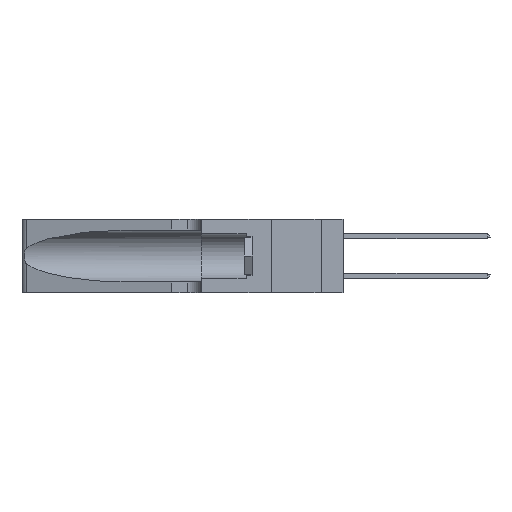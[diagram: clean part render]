
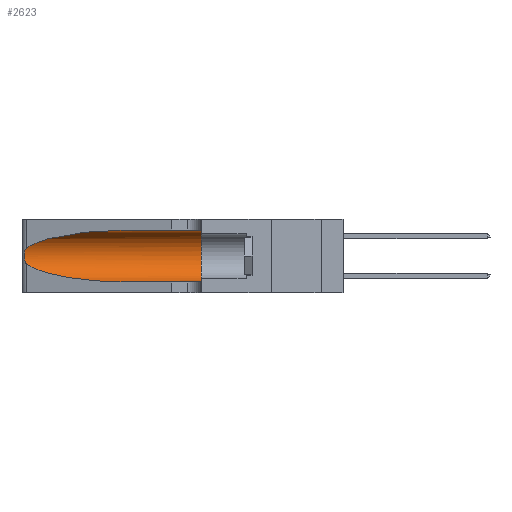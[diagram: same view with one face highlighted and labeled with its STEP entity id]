
A CAD part, left-side view. The second image highlights one B-rep face of the part: STEP entity #2623.
In plain terms, the highlighted cylindrical face has radius 3.308 mm (diameter 6.617 mm), a partial arc.
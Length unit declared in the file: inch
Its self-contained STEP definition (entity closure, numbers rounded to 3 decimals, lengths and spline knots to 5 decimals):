
#345 = B_SPLINE_CURVE_WITH_KNOTS ( 'NONE', 3,
 ( #18316, #20111, #13166, #2136, #14909, #4099, #16652, #6023, #18392, #7833, #20179, #9654, #21902, #11446 ),
 .UNSPECIFIED., .F., .F.,
 ( 4, 2, 2, 2, 2, 2, 4 ),
 ( 0., 0.00027, 0.00053, 0.00107, 0.0016, 0.00187, 0.00214 ),
 .UNSPECIFIED. ) ;
#644 = VERTEX_POINT ( 'NONE', #2025 ) ;
#1345 = DIRECTION ( 'NONE',  ( 0., -1., 0. ) ) ;
#1516 = VERTEX_POINT ( 'NONE', #12842 ) ;
#1756 = EDGE_CURVE ( 'NONE', #15566, #644, #2120, .T. ) ;
#1815 =( BOUNDED_CURVE ( )  B_SPLINE_CURVE ( 3, ( #19898, #21624, #23350, #12964 ),
 .UNSPECIFIED., .F., .F. ) 
 B_SPLINE_CURVE_WITH_KNOTS ( ( 4, 4 ),
 ( 1.5708, 2.84003 ),
 .UNSPECIFIED. ) 
 CURVE ( )  GEOMETRIC_REPRESENTATION_ITEM ( )  RATIONAL_B_SPLINE_CURVE ( ( 1., 0.87, 0.87, 1. ) ) 
 REPRESENTATION_ITEM ( '' )  );
#2025 = CARTESIAN_POINT ( 'NONE',  ( 0.1305, 0.72297, 0.05475 ) ) ;
#2120 =( BOUNDED_CURVE ( )  B_SPLINE_CURVE ( 3, ( #21580, #21173, #21603, #21093 ),
 .UNSPECIFIED., .F., .F. ) 
 B_SPLINE_CURVE_WITH_KNOTS ( ( 4, 4 ),
 ( 3.44316, 4.71239 ),
 .UNSPECIFIED. ) 
 CURVE ( )  GEOMETRIC_REPRESENTATION_ITEM ( )  RATIONAL_B_SPLINE_CURVE ( ( 1., 0.87, 0.87, 1. ) ) 
 REPRESENTATION_ITEM ( '' )  );
#2136 = CARTESIAN_POINT ( 'NONE',  ( 0.25787, 1.23484, 0.2124 ) ) ;
#2623 = ADVANCED_FACE ( 'NONE', ( #3126 ), #16939, .F. ) ;
#3126 = FACE_OUTER_BOUND ( 'NONE', #11427, .T. ) ;
#3894 = CARTESIAN_POINT ( 'NONE',  ( 0.25487, 1.22718, 0.22369 ) ) ;
#4099 = CARTESIAN_POINT ( 'NONE',  ( 0.26018, 1.23835, 0.19895 ) ) ;
#4180 = DIRECTION ( 'NONE',  ( 0., 1., 0. ) ) ;
#4981 = LINE ( 'NONE', #15289, #13988 ) ;
#5883 = EDGE_CURVE ( 'NONE', #1516, #15386, #1815, .T. ) ;
#6023 = CARTESIAN_POINT ( 'NONE',  ( 0.26075, 1.23896, 0.178 ) ) ;
#6910 = ORIENTED_EDGE ( 'NONE', *, *, #12371, .T. ) ;
#7317 = ORIENTED_EDGE ( 'NONE', *, *, #21993, .F. ) ;
#7827 = CARTESIAN_POINT ( 'NONE',  ( 0.1305, 0.35, 0.31525 ) ) ;
#7833 = CARTESIAN_POINT ( 'NONE',  ( 0.25856, 1.23593, 0.16098 ) ) ;
#8840 = ORIENTED_EDGE ( 'NONE', *, *, #1756, .T. ) ;
#9612 = LINE ( 'NONE', #22856, #13242 ) ;
#9654 = CARTESIAN_POINT ( 'NONE',  ( 0.25639, 1.23186, 0.15144 ) ) ;
#11427 = EDGE_LOOP ( 'NONE', ( #16322, #20975, #8840, #6910, #7317, #20523 ) ) ;
#11446 = CARTESIAN_POINT ( 'NONE',  ( 0.25487, 1.22718, 0.14631 ) ) ;
#12371 = EDGE_CURVE ( 'NONE', #644, #12420, #9612, .T. ) ;
#12420 = VERTEX_POINT ( 'NONE', #16020 ) ;
#12842 = CARTESIAN_POINT ( 'NONE',  ( 0.1305, 0.72297, 0.31525 ) ) ;
#12964 = CARTESIAN_POINT ( 'NONE',  ( 0.25487, 1.22718, 0.22369 ) ) ;
#13166 = CARTESIAN_POINT ( 'NONE',  ( 0.25639, 1.23184, 0.21858 ) ) ;
#13242 = VECTOR ( 'NONE', #1345, 39.37008 ) ;
#13988 = VECTOR ( 'NONE', #20493, 39.37008 ) ;
#14909 = CARTESIAN_POINT ( 'NONE',  ( 0.25854, 1.2359, 0.20912 ) ) ;
#14978 = CARTESIAN_POINT ( 'NONE',  ( 0.1305, 0.35, 0.185 ) ) ;
#15289 = CARTESIAN_POINT ( 'NONE',  ( 0.1305, 1.61858, 0.31525 ) ) ;
#15386 = VERTEX_POINT ( 'NONE', #3894 ) ;
#15527 = DIRECTION ( 'NONE',  ( 0., 0., -1. ) ) ;
#15566 = VERTEX_POINT ( 'NONE', #16829 ) ;
#16020 = CARTESIAN_POINT ( 'NONE',  ( 0.1305, 0.35, 0.05475 ) ) ;
#16162 = CARTESIAN_POINT ( 'NONE',  ( 0.1305, 1.61858, 0.185 ) ) ;
#16212 = VERTEX_POINT ( 'NONE', #7827 ) ;
#16322 = ORIENTED_EDGE ( 'NONE', *, *, #5883, .T. ) ;
#16652 = CARTESIAN_POINT ( 'NONE',  ( 0.26075, 1.23896, 0.19203 ) ) ;
#16726 = DIRECTION ( 'NONE',  ( 0., 0., 1. ) ) ;
#16829 = CARTESIAN_POINT ( 'NONE',  ( 0.25487, 1.22718, 0.14631 ) ) ;
#16939 = CYLINDRICAL_SURFACE ( 'NONE', #20843, 0.13025 ) ;
#18050 = EDGE_CURVE ( 'NONE', #15386, #15566, #345, .T. ) ;
#18316 = CARTESIAN_POINT ( 'NONE',  ( 0.25487, 1.22718, 0.22369 ) ) ;
#18392 = CARTESIAN_POINT ( 'NONE',  ( 0.26017, 1.23833, 0.17102 ) ) ;
#19898 = CARTESIAN_POINT ( 'NONE',  ( 0.1305, 0.72297, 0.31525 ) ) ;
#19998 = EDGE_CURVE ( 'NONE', #1516, #16212, #4981, .T. ) ;
#20111 = CARTESIAN_POINT ( 'NONE',  ( 0.25555, 1.22994, 0.2215 ) ) ;
#20179 = CARTESIAN_POINT ( 'NONE',  ( 0.25789, 1.23486, 0.15765 ) ) ;
#20493 = DIRECTION ( 'NONE',  ( 0., -1., 0. ) ) ;
#20523 = ORIENTED_EDGE ( 'NONE', *, *, #19998, .F. ) ;
#20843 = AXIS2_PLACEMENT_3D ( 'NONE', #16162, #22007, #15527 ) ;
#20975 = ORIENTED_EDGE ( 'NONE', *, *, #18050, .T. ) ;
#21014 = AXIS2_PLACEMENT_3D ( 'NONE', #14978, #4180, #16726 ) ;
#21093 = CARTESIAN_POINT ( 'NONE',  ( 0.1305, 0.72297, 0.05475 ) ) ;
#21173 = CARTESIAN_POINT ( 'NONE',  ( 0.2373, 1.15595, 0.08982 ) ) ;
#21580 = CARTESIAN_POINT ( 'NONE',  ( 0.25487, 1.22718, 0.14631 ) ) ;
#21603 = CARTESIAN_POINT ( 'NONE',  ( 0.18966, 0.96281, 0.05475 ) ) ;
#21624 = CARTESIAN_POINT ( 'NONE',  ( 0.18966, 0.96281, 0.31525 ) ) ;
#21770 = CIRCLE ( 'NONE', #21014, 0.13025 ) ;
#21902 = CARTESIAN_POINT ( 'NONE',  ( 0.25555, 1.22993, 0.14849 ) ) ;
#21993 = EDGE_CURVE ( 'NONE', #16212, #12420, #21770, .T. ) ;
#22007 = DIRECTION ( 'NONE',  ( 0., -1., 0. ) ) ;
#22856 = CARTESIAN_POINT ( 'NONE',  ( 0.1305, 1.61858, 0.05475 ) ) ;
#23350 = CARTESIAN_POINT ( 'NONE',  ( 0.2373, 1.15595, 0.28018 ) ) ;
